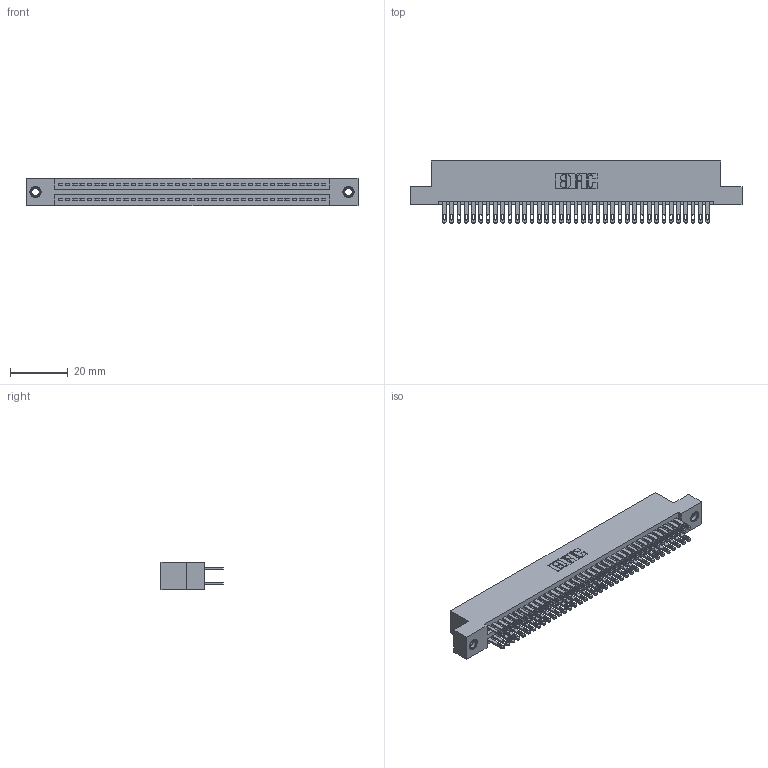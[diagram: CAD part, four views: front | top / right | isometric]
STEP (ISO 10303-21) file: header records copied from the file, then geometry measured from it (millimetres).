
FILE_DESCRIPTION (( 'STEP AP203' ), '1' );
FILE_NAME ('345-074-500-207.STEP', '2018-10-02T10:47:15', ( '' ), ( '' ), 'SwSTEP 2.0', 'SolidWorks 2016', '' );
FILE_SCHEMA (( 'CONFIG_CONTROL_DESIGN' ));
Length unit declared in the file: inch
Products named in the file (4): 345-292-001_345-293-100; 345 Part_Flush Mounting Lugs - 0.156 Dia-TI; 345-074-500-207; 345-250-001_345-250-005-103
Assembly tree (77 placements, depth 2):
  345-074-500-207
    345 Part_Flush Mounting Lugs - 0.156 Dia-TI
    345-292-001_345-293-100  x74
    345-250-001_345-250-005-103  x2
Bounding box: 115.19 x 21.51 x 9.4 mm (x, y, z)
Volume: 11355.8 mm3; surface area: 17471.5 mm2
Topology: 77 solids, 77 shells, 3590 faces, 10911 edges, 7266 vertices
Faces by surface type: plane 2110, cylinder 1464, cone 12, torus 4
Entity records: 30820 total; most frequent: CARTESIAN_POINT 5151, ORIENTED_EDGE 5078, DIRECTION 4577, EDGE_CURVE 2539, LINE 2235, VECTOR 2235, VERTEX_POINT 1688, AXIS2_PLACEMENT_3D 1171
